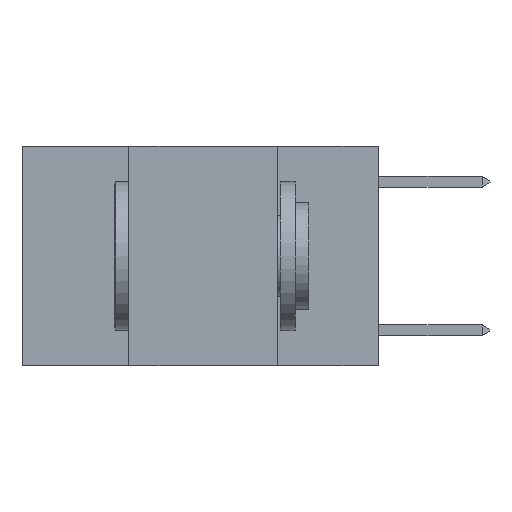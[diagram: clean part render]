
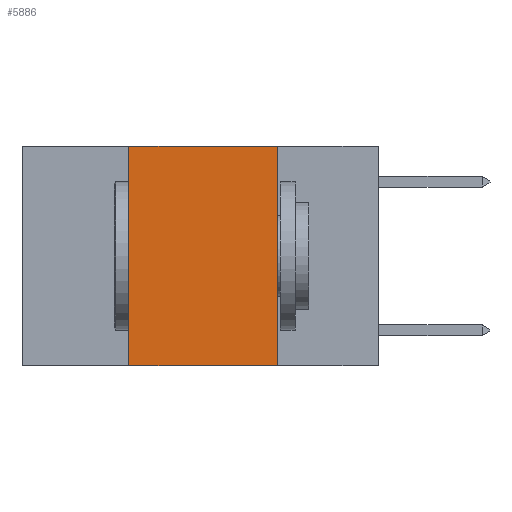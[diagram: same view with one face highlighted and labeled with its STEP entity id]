
A CAD part, left-side view. The second image highlights one B-rep face of the part: STEP entity #5886.
In plain terms, the highlighted planar face has unit normal (-1, 0, 0).
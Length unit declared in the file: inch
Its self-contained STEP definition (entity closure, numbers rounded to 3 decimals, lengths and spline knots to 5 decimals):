
#705 = VERTEX_POINT ( 'NONE', #9037 ) ;
#963 = CARTESIAN_POINT ( 'NONE',  ( 0., 0.17, -0.37 ) ) ;
#997 = CARTESIAN_POINT ( 'NONE',  ( 0., 0.42, 0. ) ) ;
#1362 = FACE_OUTER_BOUND ( 'NONE', #6701, .T. ) ;
#1461 = ORIENTED_EDGE ( 'NONE', *, *, #3662, .T. ) ;
#2098 = DIRECTION ( 'NONE',  ( 0., 0., -1. ) ) ;
#2175 = VECTOR ( 'NONE', #8884, 39.37008 ) ;
#2199 = CARTESIAN_POINT ( 'NONE',  ( 0., 0.6, -0.37 ) ) ;
#3102 = ORIENTED_EDGE ( 'NONE', *, *, #4252, .F. ) ;
#3197 = DIRECTION ( 'NONE',  ( 0., 0., 1. ) ) ;
#3198 = LINE ( 'NONE', #7663, #5781 ) ;
#3352 = ORIENTED_EDGE ( 'NONE', *, *, #5194, .F. ) ;
#3662 = EDGE_CURVE ( 'NONE', #9390, #4504, #8096, .T. ) ;
#3758 = PLANE ( 'NONE',  #6705 ) ;
#3934 = LINE ( 'NONE', #7662, #8582 ) ;
#4174 = VECTOR ( 'NONE', #5608, 39.37008 ) ;
#4252 = EDGE_CURVE ( 'NONE', #705, #4504, #3198, .T. ) ;
#4504 = VERTEX_POINT ( 'NONE', #963 ) ;
#5194 = EDGE_CURVE ( 'NONE', #9390, #8840, #3934, .T. ) ;
#5466 = LINE ( 'NONE', #7792, #4174 ) ;
#5608 = DIRECTION ( 'NONE',  ( 0., -1., 0. ) ) ;
#5781 = VECTOR ( 'NONE', #9124, 39.37008 ) ;
#5886 = ADVANCED_FACE ( 'NONE', ( #1362 ), #3758, .F. ) ;
#6617 = DIRECTION ( 'NONE',  ( 1., 0., 0. ) ) ;
#6644 = CARTESIAN_POINT ( 'NONE',  ( 0., 0.42, -0.37 ) ) ;
#6701 = EDGE_LOOP ( 'NONE', ( #3102, #7868, #3352, #1461 ) ) ;
#6705 = AXIS2_PLACEMENT_3D ( 'NONE', #6709, #6617, #2098 ) ;
#6709 = CARTESIAN_POINT ( 'NONE',  ( 0., 0.6, 0. ) ) ;
#7662 = CARTESIAN_POINT ( 'NONE',  ( 0., 0.42, 0. ) ) ;
#7663 = CARTESIAN_POINT ( 'NONE',  ( 0., 0.17, 0. ) ) ;
#7792 = CARTESIAN_POINT ( 'NONE',  ( 0., 0.6, 0. ) ) ;
#7868 = ORIENTED_EDGE ( 'NONE', *, *, #8811, .F. ) ;
#8096 = LINE ( 'NONE', #2199, #2175 ) ;
#8582 = VECTOR ( 'NONE', #3197, 39.37008 ) ;
#8811 = EDGE_CURVE ( 'NONE', #8840, #705, #5466, .T. ) ;
#8840 = VERTEX_POINT ( 'NONE', #997 ) ;
#8884 = DIRECTION ( 'NONE',  ( 0., -1., 0. ) ) ;
#9037 = CARTESIAN_POINT ( 'NONE',  ( 0., 0.17, 0. ) ) ;
#9124 = DIRECTION ( 'NONE',  ( 0., 0., -1. ) ) ;
#9390 = VERTEX_POINT ( 'NONE', #6644 ) ;
